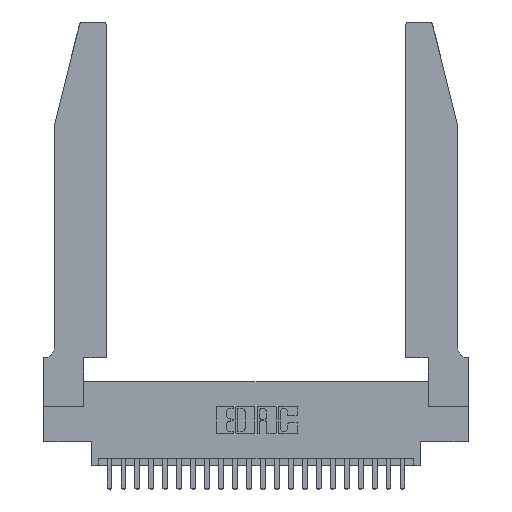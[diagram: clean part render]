
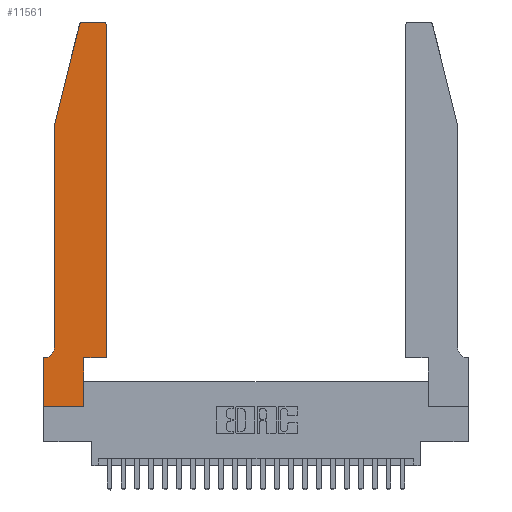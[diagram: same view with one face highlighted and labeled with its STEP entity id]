
A CAD part, top view. The second image highlights one B-rep face of the part: STEP entity #11561.
In plain terms, the highlighted planar face has unit normal (0, 0, 1).
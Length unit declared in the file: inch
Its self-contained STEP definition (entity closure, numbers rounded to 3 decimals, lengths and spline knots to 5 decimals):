
#1020 = CARTESIAN_POINT ( 'NONE',  ( 0.25487, 2.72718, 0.37 ) ) ;
#1415 = VERTEX_POINT ( 'NONE', #23026 ) ;
#1578 = AXIS2_PLACEMENT_3D ( 'NONE', #12627, #22015, #8745 ) ;
#1857 = EDGE_CURVE ( 'NONE', #22006, #3618, #20030, .T. ) ;
#2032 = CARTESIAN_POINT ( 'NONE',  ( 0.284, 2.75, 0.37 ) ) ;
#2064 = DIRECTION ( 'NONE',  ( 1., 0., 0. ) ) ;
#2346 = ORIENTED_EDGE ( 'NONE', *, *, #16499, .T. ) ;
#2395 = DIRECTION ( 'NONE',  ( 0., 1., 0. ) ) ;
#3072 = VECTOR ( 'NONE', #20749, 39.37008 ) ;
#3149 = EDGE_CURVE ( 'NONE', #21371, #22006, #7738, .T. ) ;
#3175 = EDGE_CURVE ( 'NONE', #10437, #3622, #21968, .T. ) ;
#3490 = ORIENTED_EDGE ( 'NONE', *, *, #24693, .T. ) ;
#3618 = VERTEX_POINT ( 'NONE', #21958 ) ;
#3622 = VERTEX_POINT ( 'NONE', #12323 ) ;
#3796 = CARTESIAN_POINT ( 'NONE',  ( 0.4205, 2.75, 0.37 ) ) ;
#3801 = DIRECTION ( 'NONE',  ( 1., 0., 0. ) ) ;
#4035 = ORIENTED_EDGE ( 'NONE', *, *, #4645, .T. ) ;
#4283 = LINE ( 'NONE', #8332, #13334 ) ;
#4491 = CARTESIAN_POINT ( 'NONE',  ( 0.2865, 0.35, 0.37 ) ) ;
#4645 = EDGE_CURVE ( 'NONE', #8461, #7989, #13992, .T. ) ;
#4779 = DIRECTION ( 'NONE',  ( 0., 0., 1. ) ) ;
#5431 = ORIENTED_EDGE ( 'NONE', *, *, #6745, .T. ) ;
#6745 = EDGE_CURVE ( 'NONE', #9685, #21371, #22086, .T. ) ;
#6771 = VECTOR ( 'NONE', #2395, 39.37008 ) ;
#7492 = ORIENTED_EDGE ( 'NONE', *, *, #11283, .T. ) ;
#7494 = ORIENTED_EDGE ( 'NONE', *, *, #9969, .T. ) ;
#7738 = LINE ( 'NONE', #23736, #9859 ) ;
#7989 = VERTEX_POINT ( 'NONE', #24084 ) ;
#8111 = AXIS2_PLACEMENT_3D ( 'NONE', #8484, #4779, #8649 ) ;
#8332 = CARTESIAN_POINT ( 'NONE',  ( 0.0755, 0.35, 0.37 ) ) ;
#8461 = VERTEX_POINT ( 'NONE', #14572 ) ;
#8484 = CARTESIAN_POINT ( 'NONE',  ( 0., 0.35, 0.37 ) ) ;
#8576 = ORIENTED_EDGE ( 'NONE', *, *, #14797, .T. ) ;
#8649 = DIRECTION ( 'NONE',  ( 1., 0., 0. ) ) ;
#8745 = DIRECTION ( 'NONE',  ( 1., 0., 0. ) ) ;
#9447 = CIRCLE ( 'NONE', #15361, 0.03 ) ;
#9685 = VERTEX_POINT ( 'NONE', #1020 ) ;
#9764 = CARTESIAN_POINT ( 'NONE',  ( 0.4505, 0.35, 0.37 ) ) ;
#9859 = VECTOR ( 'NONE', #18108, 39.37008 ) ;
#9969 = EDGE_CURVE ( 'NONE', #21904, #1415, #14027, .T. ) ;
#10058 = LINE ( 'NONE', #9764, #22728 ) ;
#10437 = VERTEX_POINT ( 'NONE', #10924 ) ;
#10924 = CARTESIAN_POINT ( 'NONE',  ( 0.2865, 0., 0.37 ) ) ;
#11283 = EDGE_CURVE ( 'NONE', #3622, #8461, #10058, .T. ) ;
#11350 = CARTESIAN_POINT ( 'NONE',  ( 0.0055, 0.42, 0.37 ) ) ;
#11434 = CARTESIAN_POINT ( 'NONE',  ( 0., 0., 0.37 ) ) ;
#11561 = ADVANCED_FACE ( 'NONE', ( #16962 ), #23772, .T. ) ;
#11758 = DIRECTION ( 'NONE',  ( 0., 0., 1. ) ) ;
#11793 = DIRECTION ( 'NONE',  ( 0., -1., 0. ) ) ;
#12323 = CARTESIAN_POINT ( 'NONE',  ( 0.2865, 0.35, 0.37 ) ) ;
#12334 = CARTESIAN_POINT ( 'NONE',  ( 0.0755, 2., 0.37 ) ) ;
#12627 = CARTESIAN_POINT ( 'NONE',  ( 0.4205, 2.72, 0.37 ) ) ;
#12801 = AXIS2_PLACEMENT_3D ( 'NONE', #11350, #13287, #24587 ) ;
#12965 = ORIENTED_EDGE ( 'NONE', *, *, #3175, .T. ) ;
#13287 = DIRECTION ( 'NONE',  ( 0., 0., -1. ) ) ;
#13334 = VECTOR ( 'NONE', #15923, 39.37008 ) ;
#13474 = VECTOR ( 'NONE', #16211, 39.37008 ) ;
#13746 = CARTESIAN_POINT ( 'NONE',  ( 0.284, 2.72, 0.37 ) ) ;
#13992 = LINE ( 'NONE', #16663, #6771 ) ;
#14027 = LINE ( 'NONE', #17353, #17354 ) ;
#14254 = VERTEX_POINT ( 'NONE', #2032 ) ;
#14390 = VECTOR ( 'NONE', #2064, 39.37008 ) ;
#14572 = CARTESIAN_POINT ( 'NONE',  ( 0.4505, 0.35, 0.37 ) ) ;
#14797 = EDGE_CURVE ( 'NONE', #22105, #14254, #22121, .T. ) ;
#15361 = AXIS2_PLACEMENT_3D ( 'NONE', #13746, #11758, #3801 ) ;
#15368 = ORIENTED_EDGE ( 'NONE', *, *, #20305, .T. ) ;
#15923 = DIRECTION ( 'NONE',  ( -1., 0., 0. ) ) ;
#16211 = DIRECTION ( 'NONE',  ( 0., 1., 0. ) ) ;
#16291 = DIRECTION ( 'NONE',  ( -0.239, -0.971, 0. ) ) ;
#16499 = EDGE_CURVE ( 'NONE', #7989, #22105, #22896, .T. ) ;
#16663 = CARTESIAN_POINT ( 'NONE',  ( 0.4505, 0.35, 0.37 ) ) ;
#16962 = FACE_OUTER_BOUND ( 'NONE', #17017, .T. ) ;
#17017 = EDGE_LOOP ( 'NONE', ( #8576, #15368, #5431, #17763, #21987, #20986, #7494, #3490, #12965, #7492, #4035, #2346 ) ) ;
#17183 = DIRECTION ( 'NONE',  ( 1., 0., 0. ) ) ;
#17218 = CARTESIAN_POINT ( 'NONE',  ( 0.0755, 0.42, 0.37 ) ) ;
#17353 = CARTESIAN_POINT ( 'NONE',  ( 0., 0., 0.37 ) ) ;
#17354 = VECTOR ( 'NONE', #11793, 39.37008 ) ;
#17763 = ORIENTED_EDGE ( 'NONE', *, *, #3149, .T. ) ;
#18108 = DIRECTION ( 'NONE',  ( 0., -1., 0. ) ) ;
#18610 = CARTESIAN_POINT ( 'NONE',  ( 0., 0.35, 0.37 ) ) ;
#18824 = CARTESIAN_POINT ( 'NONE',  ( 0.2605, 2.75, 0.37 ) ) ;
#19062 = VECTOR ( 'NONE', #16291, 39.37008 ) ;
#20030 = CIRCLE ( 'NONE', #12801, 0.07 ) ;
#20305 = EDGE_CURVE ( 'NONE', #14254, #9685, #9447, .T. ) ;
#20337 = CARTESIAN_POINT ( 'NONE',  ( 0.0755, 2., 0.37 ) ) ;
#20749 = DIRECTION ( 'NONE',  ( -1., 0., 0. ) ) ;
#20986 = ORIENTED_EDGE ( 'NONE', *, *, #21208, .T. ) ;
#21208 = EDGE_CURVE ( 'NONE', #3618, #21904, #4283, .T. ) ;
#21371 = VERTEX_POINT ( 'NONE', #20337 ) ;
#21904 = VERTEX_POINT ( 'NONE', #18610 ) ;
#21958 = CARTESIAN_POINT ( 'NONE',  ( 0.0055, 0.35, 0.37 ) ) ;
#21968 = LINE ( 'NONE', #4491, #13474 ) ;
#21987 = ORIENTED_EDGE ( 'NONE', *, *, #1857, .T. ) ;
#22006 = VERTEX_POINT ( 'NONE', #17218 ) ;
#22015 = DIRECTION ( 'NONE',  ( 0., 0., 1. ) ) ;
#22086 = LINE ( 'NONE', #12334, #19062 ) ;
#22105 = VERTEX_POINT ( 'NONE', #3796 ) ;
#22121 = LINE ( 'NONE', #18824, #3072 ) ;
#22728 = VECTOR ( 'NONE', #17183, 39.37008 ) ;
#22896 = CIRCLE ( 'NONE', #1578, 0.03 ) ;
#23026 = CARTESIAN_POINT ( 'NONE',  ( 0., 0., 0.37 ) ) ;
#23736 = CARTESIAN_POINT ( 'NONE',  ( 0.0755, 2., 0.37 ) ) ;
#23772 = PLANE ( 'NONE',  #8111 ) ;
#24084 = CARTESIAN_POINT ( 'NONE',  ( 0.4505, 2.72, 0.37 ) ) ;
#24587 = DIRECTION ( 'NONE',  ( -1., 0., 0. ) ) ;
#24633 = LINE ( 'NONE', #11434, #14390 ) ;
#24693 = EDGE_CURVE ( 'NONE', #1415, #10437, #24633, .T. ) ;
